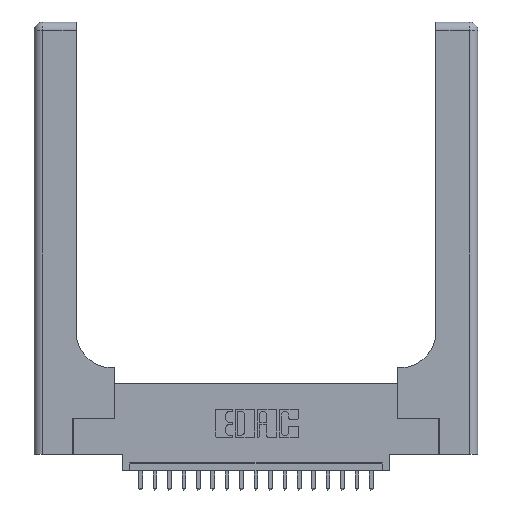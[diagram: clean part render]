
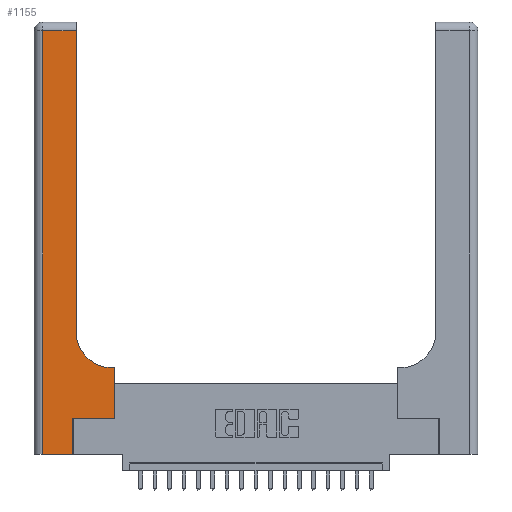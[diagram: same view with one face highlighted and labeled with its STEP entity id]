
A CAD part, top view. The second image highlights one B-rep face of the part: STEP entity #1155.
In plain terms, the highlighted planar face has unit normal (0, 0, 1).
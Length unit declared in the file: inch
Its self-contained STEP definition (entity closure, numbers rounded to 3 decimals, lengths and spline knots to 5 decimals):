
#97 = ORIENTED_EDGE ( 'NONE', *, *, #2924, .T. ) ;
#278 = CARTESIAN_POINT ( 'NONE',  ( 0.2915, 3., 0.37 ) ) ;
#398 = VECTOR ( 'NONE', #6309, 39.37008 ) ;
#812 = LINE ( 'NONE', #19981, #4176 ) ;
#1155 = ADVANCED_FACE ( 'NONE', ( #7210 ), #19163, .F. ) ;
#1241 = CARTESIAN_POINT ( 'NONE',  ( 0.2915, 0.6, 0.37 ) ) ;
#1962 = CARTESIAN_POINT ( 'NONE',  ( 0.5415, 0.6, 0.37 ) ) ;
#2291 = DIRECTION ( 'NONE',  ( 0., 0., -1. ) ) ;
#2475 = LINE ( 'NONE', #1241, #398 ) ;
#2512 = CARTESIAN_POINT ( 'NONE',  ( 0.5415, 0.85, 0.37 ) ) ;
#2795 = ORIENTED_EDGE ( 'NONE', *, *, #17058, .T. ) ;
#2924 = EDGE_CURVE ( 'NONE', #7853, #15218, #20714, .T. ) ;
#3629 = AXIS2_PLACEMENT_3D ( 'NONE', #4356, #20900, #9277 ) ;
#3728 = EDGE_CURVE ( 'NONE', #8201, #5131, #17925, .T. ) ;
#3883 = VERTEX_POINT ( 'NONE', #17641 ) ;
#4176 = VECTOR ( 'NONE', #16439, 39.37008 ) ;
#4295 = ORIENTED_EDGE ( 'NONE', *, *, #13255, .T. ) ;
#4356 = CARTESIAN_POINT ( 'NONE',  ( 0., 3., 0.37 ) ) ;
#4464 = CARTESIAN_POINT ( 'NONE',  ( 0.06, 3., 0.37 ) ) ;
#4490 = CARTESIAN_POINT ( 'NONE',  ( 0.06, 0., 0.37 ) ) ;
#4625 = VERTEX_POINT ( 'NONE', #1962 ) ;
#4762 = ORIENTED_EDGE ( 'NONE', *, *, #3728, .T. ) ;
#4965 = CARTESIAN_POINT ( 'NONE',  ( 0.269, 0.25, 0.37 ) ) ;
#5131 = VERTEX_POINT ( 'NONE', #17981 ) ;
#5714 = DIRECTION ( 'NONE',  ( 1., 0., 0. ) ) ;
#5859 = EDGE_CURVE ( 'NONE', #5131, #4625, #2475, .T. ) ;
#6226 = VECTOR ( 'NONE', #19706, 39.37008 ) ;
#6309 = DIRECTION ( 'NONE',  ( -1., 0., 0. ) ) ;
#6317 = CARTESIAN_POINT ( 'NONE',  ( 0.269, 0.25, 0.37 ) ) ;
#7084 = AXIS2_PLACEMENT_3D ( 'NONE', #2512, #2291, #5714 ) ;
#7210 = FACE_OUTER_BOUND ( 'NONE', #20105, .T. ) ;
#7478 = VERTEX_POINT ( 'NONE', #20505 ) ;
#7739 = CARTESIAN_POINT ( 'NONE',  ( 0.2915, 0.85, 0.37 ) ) ;
#7785 = VERTEX_POINT ( 'NONE', #7739 ) ;
#7853 = VERTEX_POINT ( 'NONE', #18004 ) ;
#8038 = LINE ( 'NONE', #4965, #20282 ) ;
#8201 = VERTEX_POINT ( 'NONE', #20736 ) ;
#8916 = ORIENTED_EDGE ( 'NONE', *, *, #15364, .T. ) ;
#9166 = EDGE_CURVE ( 'NONE', #15218, #7478, #812, .T. ) ;
#9277 = DIRECTION ( 'NONE',  ( -1., 0., 0. ) ) ;
#9442 = VECTOR ( 'NONE', #12097, 39.37008 ) ;
#9826 = CARTESIAN_POINT ( 'NONE',  ( 0.269, 0., 0.37 ) ) ;
#9947 = DIRECTION ( 'NONE',  ( 0., 1., 0. ) ) ;
#10706 = ORIENTED_EDGE ( 'NONE', *, *, #5859, .T. ) ;
#11692 = ORIENTED_EDGE ( 'NONE', *, *, #9166, .T. ) ;
#11701 = VERTEX_POINT ( 'NONE', #6317 ) ;
#11981 = DIRECTION ( 'NONE',  ( 0., 1., 0. ) ) ;
#12097 = DIRECTION ( 'NONE',  ( -1., 0., 0. ) ) ;
#12654 = EDGE_CURVE ( 'NONE', #4625, #7785, #17020, .T. ) ;
#13255 = EDGE_CURVE ( 'NONE', #3883, #7853, #15194, .T. ) ;
#13313 = VECTOR ( 'NONE', #11981, 39.37008 ) ;
#13537 = LINE ( 'NONE', #9826, #6226 ) ;
#13700 = CARTESIAN_POINT ( 'NONE',  ( 0., 2.94, 0.37 ) ) ;
#15025 = VECTOR ( 'NONE', #16064, 39.37008 ) ;
#15194 = LINE ( 'NONE', #13700, #9442 ) ;
#15218 = VERTEX_POINT ( 'NONE', #4490 ) ;
#15364 = EDGE_CURVE ( 'NONE', #7785, #3883, #15400, .T. ) ;
#15400 = LINE ( 'NONE', #278, #13313 ) ;
#16064 = DIRECTION ( 'NONE',  ( 0., -1., 0. ) ) ;
#16439 = DIRECTION ( 'NONE',  ( 1., 0., 0. ) ) ;
#17020 = CIRCLE ( 'NONE', #7084, 0.25 ) ;
#17058 = EDGE_CURVE ( 'NONE', #11701, #8201, #8038, .T. ) ;
#17400 = ORIENTED_EDGE ( 'NONE', *, *, #17918, .T. ) ;
#17404 = VECTOR ( 'NONE', #9947, 39.37008 ) ;
#17641 = CARTESIAN_POINT ( 'NONE',  ( 0.2915, 2.94, 0.37 ) ) ;
#17918 = EDGE_CURVE ( 'NONE', #7478, #11701, #13537, .T. ) ;
#17925 = LINE ( 'NONE', #17958, #17404 ) ;
#17958 = CARTESIAN_POINT ( 'NONE',  ( 0.5585, 0.25, 0.37 ) ) ;
#17981 = CARTESIAN_POINT ( 'NONE',  ( 0.5585, 0.6, 0.37 ) ) ;
#18004 = CARTESIAN_POINT ( 'NONE',  ( 0.06, 2.94, 0.37 ) ) ;
#18471 = DIRECTION ( 'NONE',  ( 1., 0., 0. ) ) ;
#19163 = PLANE ( 'NONE',  #3629 ) ;
#19706 = DIRECTION ( 'NONE',  ( 0., 1., 0. ) ) ;
#19981 = CARTESIAN_POINT ( 'NONE',  ( 0., 0., 0.37 ) ) ;
#20105 = EDGE_LOOP ( 'NONE', ( #8916, #4295, #97, #11692, #17400, #2795, #4762, #10706, #20519 ) ) ;
#20282 = VECTOR ( 'NONE', #18471, 39.37008 ) ;
#20505 = CARTESIAN_POINT ( 'NONE',  ( 0.269, 0., 0.37 ) ) ;
#20519 = ORIENTED_EDGE ( 'NONE', *, *, #12654, .T. ) ;
#20714 = LINE ( 'NONE', #4464, #15025 ) ;
#20736 = CARTESIAN_POINT ( 'NONE',  ( 0.5585, 0.25, 0.37 ) ) ;
#20900 = DIRECTION ( 'NONE',  ( 0., 0., -1. ) ) ;
